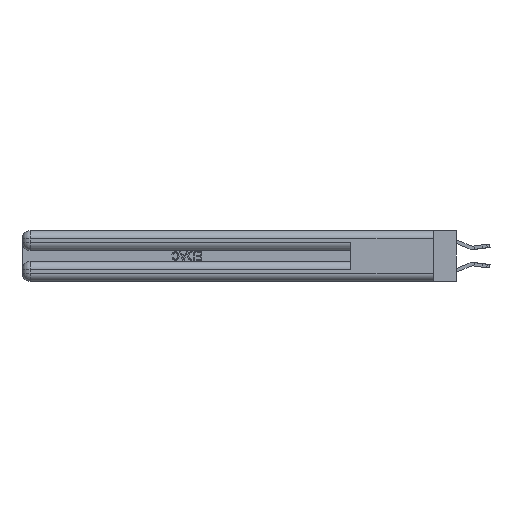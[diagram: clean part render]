
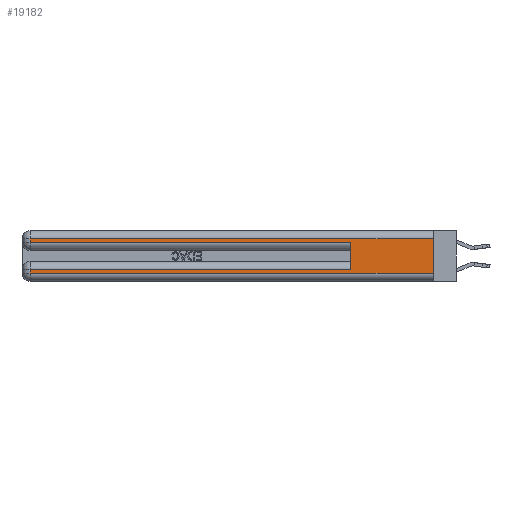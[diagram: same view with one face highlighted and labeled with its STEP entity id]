
A CAD part, left-side view. The second image highlights one B-rep face of the part: STEP entity #19182.
In plain terms, the highlighted planar face has unit normal (-1, 0, 0).
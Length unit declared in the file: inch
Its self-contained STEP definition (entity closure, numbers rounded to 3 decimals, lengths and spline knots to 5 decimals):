
#160 = VECTOR ( 'NONE', #16644, 39.37008 ) ;
#1655 = VERTEX_POINT ( 'NONE', #3863 ) ;
#2382 = DIRECTION ( 'NONE',  ( 0., 0., -1. ) ) ;
#2981 = ORIENTED_EDGE ( 'NONE', *, *, #4615, .T. ) ;
#3003 = EDGE_CURVE ( 'NONE', #20353, #24475, #21745, .T. ) ;
#3015 = VERTEX_POINT ( 'NONE', #18205 ) ;
#3357 = EDGE_CURVE ( 'NONE', #27713, #10791, #21321, .T. ) ;
#3863 = CARTESIAN_POINT ( 'NONE',  ( 0., 2.94, 0.285 ) ) ;
#4245 = CARTESIAN_POINT ( 'NONE',  ( 0., 0.6, 0.285 ) ) ;
#4615 = EDGE_CURVE ( 'NONE', #26610, #27713, #17411, .T. ) ;
#6233 = ORIENTED_EDGE ( 'NONE', *, *, #3003, .T. ) ;
#7314 = CARTESIAN_POINT ( 'NONE',  ( 0., 2.94, 0.06 ) ) ;
#7568 = CARTESIAN_POINT ( 'NONE',  ( 0., 2.94, 0.37 ) ) ;
#8404 = LINE ( 'NONE', #17775, #26114 ) ;
#8447 = CARTESIAN_POINT ( 'NONE',  ( 0., 0., 0.31 ) ) ;
#9860 = ORIENTED_EDGE ( 'NONE', *, *, #13911, .F. ) ;
#10631 = CARTESIAN_POINT ( 'NONE',  ( 0., 0., 0.285 ) ) ;
#10791 = VERTEX_POINT ( 'NONE', #7314 ) ;
#11262 = DIRECTION ( 'NONE',  ( 1., 0., 0. ) ) ;
#12311 = DIRECTION ( 'NONE',  ( 0., -1., 0. ) ) ;
#13042 = ORIENTED_EDGE ( 'NONE', *, *, #26506, .T. ) ;
#13802 = DIRECTION ( 'NONE',  ( 0., 0., -1. ) ) ;
#13911 = EDGE_CURVE ( 'NONE', #20353, #3015, #14316, .T. ) ;
#13961 = PLANE ( 'NONE',  #17165 ) ;
#14316 = LINE ( 'NONE', #23514, #29526 ) ;
#14590 = LINE ( 'NONE', #24238, #16448 ) ;
#14697 = ORIENTED_EDGE ( 'NONE', *, *, #20058, .T. ) ;
#14950 = DIRECTION ( 'NONE',  ( 0., 1., 0. ) ) ;
#15161 = LINE ( 'NONE', #10631, #16555 ) ;
#15937 = CARTESIAN_POINT ( 'NONE',  ( 0., 0., 0.31 ) ) ;
#16054 = EDGE_CURVE ( 'NONE', #1655, #29135, #15161, .T. ) ;
#16197 = VECTOR ( 'NONE', #29195, 39.37008 ) ;
#16448 = VECTOR ( 'NONE', #12311, 39.37008 ) ;
#16555 = VECTOR ( 'NONE', #17125, 39.37008 ) ;
#16644 = DIRECTION ( 'NONE',  ( 0., 0., -1. ) ) ;
#17125 = DIRECTION ( 'NONE',  ( 0., -1., 0. ) ) ;
#17165 = AXIS2_PLACEMENT_3D ( 'NONE', #27860, #11262, #13802 ) ;
#17411 = LINE ( 'NONE', #24479, #16197 ) ;
#17775 = CARTESIAN_POINT ( 'NONE',  ( 0., 0.6, 0.145 ) ) ;
#17902 = CARTESIAN_POINT ( 'NONE',  ( 0., 0.6, 0.085 ) ) ;
#18202 = ORIENTED_EDGE ( 'NONE', *, *, #28653, .F. ) ;
#18205 = CARTESIAN_POINT ( 'NONE',  ( 0., 0., 0.06 ) ) ;
#18244 = ORIENTED_EDGE ( 'NONE', *, *, #16054, .T. ) ;
#18635 = FACE_OUTER_BOUND ( 'NONE', #19194, .T. ) ;
#19160 = VECTOR ( 'NONE', #14950, 39.37008 ) ;
#19182 = ADVANCED_FACE ( 'NONE', ( #18635 ), #13961, .F. ) ;
#19194 = EDGE_LOOP ( 'NONE', ( #9860, #6233, #14697, #18244, #18202, #2981, #25790, #13042 ) ) ;
#19621 = VECTOR ( 'NONE', #25225, 39.37008 ) ;
#20058 = EDGE_CURVE ( 'NONE', #24475, #1655, #29507, .T. ) ;
#20353 = VERTEX_POINT ( 'NONE', #8447 ) ;
#21321 = LINE ( 'NONE', #7568, #160 ) ;
#21745 = LINE ( 'NONE', #15937, #19160 ) ;
#23514 = CARTESIAN_POINT ( 'NONE',  ( 0., 0., 0.37 ) ) ;
#23663 = CARTESIAN_POINT ( 'NONE',  ( 0., 2.94, 0.31 ) ) ;
#24238 = CARTESIAN_POINT ( 'NONE',  ( 0., 0., 0.06 ) ) ;
#24475 = VERTEX_POINT ( 'NONE', #23663 ) ;
#24479 = CARTESIAN_POINT ( 'NONE',  ( 0., 0., 0.085 ) ) ;
#25225 = DIRECTION ( 'NONE',  ( 0., 0., -1. ) ) ;
#25790 = ORIENTED_EDGE ( 'NONE', *, *, #3357, .T. ) ;
#25797 = CARTESIAN_POINT ( 'NONE',  ( 0., 2.94, 0.085 ) ) ;
#26114 = VECTOR ( 'NONE', #26690, 39.37008 ) ;
#26506 = EDGE_CURVE ( 'NONE', #10791, #3015, #14590, .T. ) ;
#26610 = VERTEX_POINT ( 'NONE', #17902 ) ;
#26690 = DIRECTION ( 'NONE',  ( 0., 0., 1. ) ) ;
#27713 = VERTEX_POINT ( 'NONE', #25797 ) ;
#27860 = CARTESIAN_POINT ( 'NONE',  ( 0., 0., 0.37 ) ) ;
#28653 = EDGE_CURVE ( 'NONE', #26610, #29135, #8404, .T. ) ;
#29135 = VERTEX_POINT ( 'NONE', #4245 ) ;
#29195 = DIRECTION ( 'NONE',  ( 0., 1., 0. ) ) ;
#29354 = CARTESIAN_POINT ( 'NONE',  ( 0., 2.94, 0.37 ) ) ;
#29507 = LINE ( 'NONE', #29354, #19621 ) ;
#29526 = VECTOR ( 'NONE', #2382, 39.37008 ) ;
